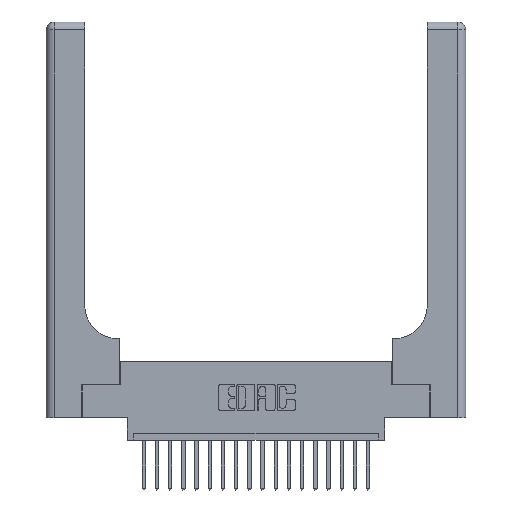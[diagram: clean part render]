
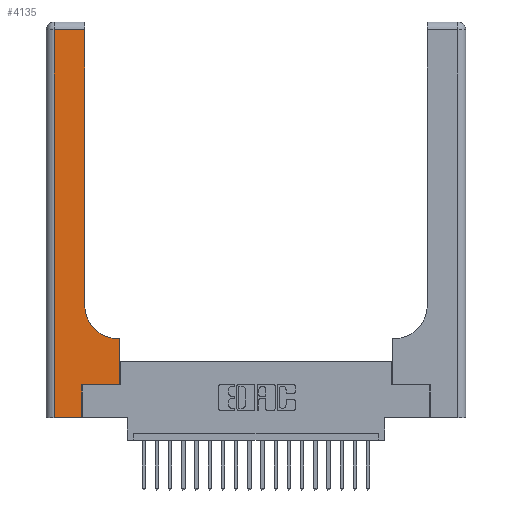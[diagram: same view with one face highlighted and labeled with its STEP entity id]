
A CAD part, top view. The second image highlights one B-rep face of the part: STEP entity #4135.
In plain terms, the highlighted planar face has unit normal (0, 0, 1).
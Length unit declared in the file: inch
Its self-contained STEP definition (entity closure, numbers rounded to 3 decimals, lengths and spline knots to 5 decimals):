
#633 = VECTOR ( 'NONE', #6225, 39.37008 ) ;
#821 = CARTESIAN_POINT ( 'NONE',  ( 0.2915, 0.6, 0.37 ) ) ;
#1030 = CARTESIAN_POINT ( 'NONE',  ( 0.2915, 3., 0.37 ) ) ;
#1332 = VERTEX_POINT ( 'NONE', #7815 ) ;
#1921 = VERTEX_POINT ( 'NONE', #6371 ) ;
#2045 = ORIENTED_EDGE ( 'NONE', *, *, #4997, .T. ) ;
#3019 = FACE_OUTER_BOUND ( 'NONE', #15354, .T. ) ;
#3390 = VERTEX_POINT ( 'NONE', #10264 ) ;
#3399 = VERTEX_POINT ( 'NONE', #15399 ) ;
#3785 = LINE ( 'NONE', #821, #4064 ) ;
#3966 = EDGE_CURVE ( 'NONE', #12725, #17241, #17715, .T. ) ;
#4064 = VECTOR ( 'NONE', #5973, 39.37008 ) ;
#4070 = ORIENTED_EDGE ( 'NONE', *, *, #8511, .T. ) ;
#4071 = AXIS2_PLACEMENT_3D ( 'NONE', #11582, #5299, #15560 ) ;
#4135 = ADVANCED_FACE ( 'NONE', ( #3019 ), #9826, .F. ) ;
#4997 = EDGE_CURVE ( 'NONE', #3390, #13967, #20843, .T. ) ;
#5034 = ORIENTED_EDGE ( 'NONE', *, *, #3966, .T. ) ;
#5103 = LINE ( 'NONE', #8421, #7003 ) ;
#5299 = DIRECTION ( 'NONE',  ( 0., 0., -1. ) ) ;
#5316 = ORIENTED_EDGE ( 'NONE', *, *, #14110, .T. ) ;
#5340 = VECTOR ( 'NONE', #9801, 39.37008 ) ;
#5491 = ORIENTED_EDGE ( 'NONE', *, *, #14672, .T. ) ;
#5973 = DIRECTION ( 'NONE',  ( -1., 0., 0. ) ) ;
#6225 = DIRECTION ( 'NONE',  ( 1., 0., 0. ) ) ;
#6371 = CARTESIAN_POINT ( 'NONE',  ( 0.5585, 0.6, 0.37 ) ) ;
#6769 = DIRECTION ( 'NONE',  ( -1., 0., 0. ) ) ;
#6893 = DIRECTION ( 'NONE',  ( 0., 1., 0. ) ) ;
#7003 = VECTOR ( 'NONE', #11697, 39.37008 ) ;
#7017 = VECTOR ( 'NONE', #20445, 39.37008 ) ;
#7067 = VECTOR ( 'NONE', #6769, 39.37008 ) ;
#7815 = CARTESIAN_POINT ( 'NONE',  ( 0.2915, 2.94, 0.37 ) ) ;
#7972 = CARTESIAN_POINT ( 'NONE',  ( 0., 2.94, 0.37 ) ) ;
#8421 = CARTESIAN_POINT ( 'NONE',  ( 0.06, 3., 0.37 ) ) ;
#8511 = EDGE_CURVE ( 'NONE', #1332, #18827, #11654, .T. ) ;
#9380 = CARTESIAN_POINT ( 'NONE',  ( 0., 0., 0.37 ) ) ;
#9387 = VECTOR ( 'NONE', #6893, 39.37008 ) ;
#9801 = DIRECTION ( 'NONE',  ( 0., 1., 0. ) ) ;
#9826 = PLANE ( 'NONE',  #4071 ) ;
#9927 = LINE ( 'NONE', #1030, #5340 ) ;
#10264 = CARTESIAN_POINT ( 'NONE',  ( 0.06, 0., 0.37 ) ) ;
#11384 = DIRECTION ( 'NONE',  ( 0., 0., -1. ) ) ;
#11503 = CIRCLE ( 'NONE', #19327, 0.25 ) ;
#11582 = CARTESIAN_POINT ( 'NONE',  ( 0., 3., 0.37 ) ) ;
#11654 = LINE ( 'NONE', #7972, #7067 ) ;
#11697 = DIRECTION ( 'NONE',  ( 0., -1., 0. ) ) ;
#11835 = EDGE_CURVE ( 'NONE', #15731, #3399, #11503, .T. ) ;
#12307 = ORIENTED_EDGE ( 'NONE', *, *, #15185, .T. ) ;
#12630 = LINE ( 'NONE', #20779, #21368 ) ;
#12725 = VERTEX_POINT ( 'NONE', #21088 ) ;
#13967 = VERTEX_POINT ( 'NONE', #21931 ) ;
#14110 = EDGE_CURVE ( 'NONE', #17241, #1921, #19516, .T. ) ;
#14429 = ORIENTED_EDGE ( 'NONE', *, *, #11835, .T. ) ;
#14672 = EDGE_CURVE ( 'NONE', #18827, #3390, #5103, .T. ) ;
#14977 = CARTESIAN_POINT ( 'NONE',  ( 0.269, 0.25, 0.37 ) ) ;
#15185 = EDGE_CURVE ( 'NONE', #13967, #12725, #12630, .T. ) ;
#15354 = EDGE_LOOP ( 'NONE', ( #20693, #4070, #5491, #2045, #12307, #5034, #5316, #16088, #14429 ) ) ;
#15399 = CARTESIAN_POINT ( 'NONE',  ( 0.2915, 0.85, 0.37 ) ) ;
#15560 = DIRECTION ( 'NONE',  ( -1., 0., 0. ) ) ;
#15642 = EDGE_CURVE ( 'NONE', #3399, #1332, #9927, .T. ) ;
#15670 = DIRECTION ( 'NONE',  ( 0., 1., 0. ) ) ;
#15731 = VERTEX_POINT ( 'NONE', #18259 ) ;
#16088 = ORIENTED_EDGE ( 'NONE', *, *, #19964, .T. ) ;
#16535 = DIRECTION ( 'NONE',  ( 1., 0., 0. ) ) ;
#17070 = CARTESIAN_POINT ( 'NONE',  ( 0.5585, 0.25, 0.37 ) ) ;
#17241 = VERTEX_POINT ( 'NONE', #19595 ) ;
#17715 = LINE ( 'NONE', #14977, #633 ) ;
#18259 = CARTESIAN_POINT ( 'NONE',  ( 0.5415, 0.6, 0.37 ) ) ;
#18827 = VERTEX_POINT ( 'NONE', #21374 ) ;
#19327 = AXIS2_PLACEMENT_3D ( 'NONE', #21526, #11384, #16535 ) ;
#19516 = LINE ( 'NONE', #17070, #9387 ) ;
#19595 = CARTESIAN_POINT ( 'NONE',  ( 0.5585, 0.25, 0.37 ) ) ;
#19964 = EDGE_CURVE ( 'NONE', #1921, #15731, #3785, .T. ) ;
#20445 = DIRECTION ( 'NONE',  ( 1., 0., 0. ) ) ;
#20693 = ORIENTED_EDGE ( 'NONE', *, *, #15642, .T. ) ;
#20779 = CARTESIAN_POINT ( 'NONE',  ( 0.269, 0., 0.37 ) ) ;
#20843 = LINE ( 'NONE', #9380, #7017 ) ;
#21088 = CARTESIAN_POINT ( 'NONE',  ( 0.269, 0.25, 0.37 ) ) ;
#21368 = VECTOR ( 'NONE', #15670, 39.37008 ) ;
#21374 = CARTESIAN_POINT ( 'NONE',  ( 0.06, 2.94, 0.37 ) ) ;
#21526 = CARTESIAN_POINT ( 'NONE',  ( 0.5415, 0.85, 0.37 ) ) ;
#21931 = CARTESIAN_POINT ( 'NONE',  ( 0.269, 0., 0.37 ) ) ;
